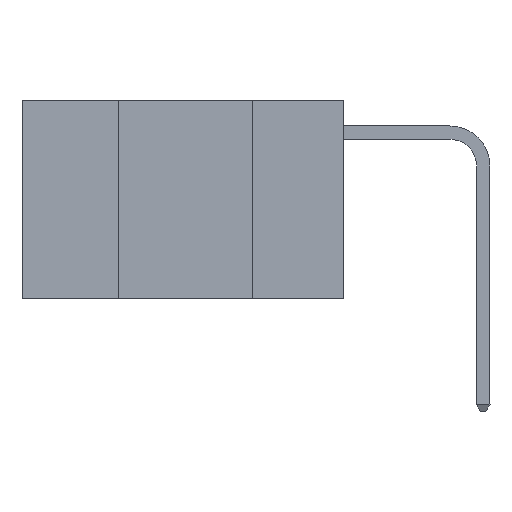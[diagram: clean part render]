
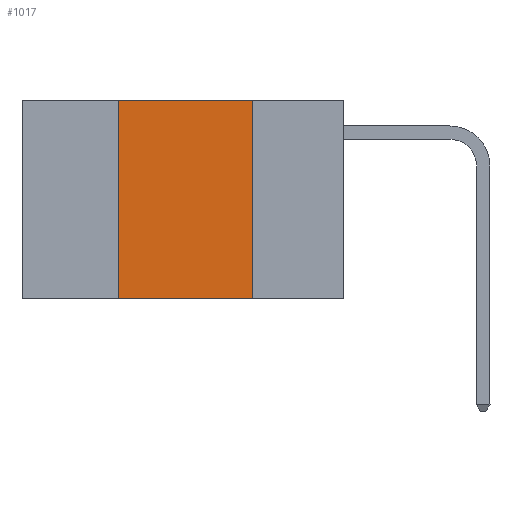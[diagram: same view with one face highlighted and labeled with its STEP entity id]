
A CAD part, left-side view. The second image highlights one B-rep face of the part: STEP entity #1017.
In plain terms, the highlighted planar face has unit normal (-1, 0, 0).
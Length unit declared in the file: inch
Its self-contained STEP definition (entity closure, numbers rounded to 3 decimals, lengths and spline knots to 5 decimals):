
#673 = ORIENTED_EDGE ( 'NONE', *, *, #3448, .F. ) ;
#968 = EDGE_CURVE ( 'NONE', #1902, #14417, #13548, .T. ) ;
#1017 = ADVANCED_FACE ( 'NONE', ( #9887 ), #10258, .F. ) ;
#1463 = VECTOR ( 'NONE', #7913, 39.37008 ) ;
#1902 = VERTEX_POINT ( 'NONE', #14021 ) ;
#2383 = LINE ( 'NONE', #5336, #5076 ) ;
#2518 = CARTESIAN_POINT ( 'NONE',  ( 0., 0.42, 0. ) ) ;
#3425 = DIRECTION ( 'NONE',  ( 1., 0., 0. ) ) ;
#3448 = EDGE_CURVE ( 'NONE', #1902, #10002, #7911, .T. ) ;
#4842 = VECTOR ( 'NONE', #9116, 39.37008 ) ;
#5076 = VECTOR ( 'NONE', #11002, 39.37008 ) ;
#5336 = CARTESIAN_POINT ( 'NONE',  ( 0., 0.6, 0. ) ) ;
#6303 = ORIENTED_EDGE ( 'NONE', *, *, #12049, .F. ) ;
#6387 = ORIENTED_EDGE ( 'NONE', *, *, #968, .T. ) ;
#7552 = LINE ( 'NONE', #14321, #13147 ) ;
#7606 = EDGE_CURVE ( 'NONE', #10962, #14417, #7552, .T. ) ;
#7911 = LINE ( 'NONE', #14645, #4842 ) ;
#7913 = DIRECTION ( 'NONE',  ( 0., -1., 0. ) ) ;
#7993 = EDGE_LOOP ( 'NONE', ( #13524, #6303, #673, #6387 ) ) ;
#8008 = CARTESIAN_POINT ( 'NONE',  ( 0., 0.6, 0. ) ) ;
#8070 = CARTESIAN_POINT ( 'NONE',  ( 0., 0.17, -0.37 ) ) ;
#9116 = DIRECTION ( 'NONE',  ( 0., 0., 1. ) ) ;
#9887 = FACE_OUTER_BOUND ( 'NONE', #7993, .T. ) ;
#10002 = VERTEX_POINT ( 'NONE', #2518 ) ;
#10258 = PLANE ( 'NONE',  #10731 ) ;
#10731 = AXIS2_PLACEMENT_3D ( 'NONE', #8008, #3425, #11369 ) ;
#10962 = VERTEX_POINT ( 'NONE', #14574 ) ;
#11002 = DIRECTION ( 'NONE',  ( 0., -1., 0. ) ) ;
#11016 = DIRECTION ( 'NONE',  ( 0., 0., -1. ) ) ;
#11369 = DIRECTION ( 'NONE',  ( 0., 0., -1. ) ) ;
#12049 = EDGE_CURVE ( 'NONE', #10002, #10962, #2383, .T. ) ;
#13147 = VECTOR ( 'NONE', #11016, 39.37008 ) ;
#13477 = CARTESIAN_POINT ( 'NONE',  ( 0., 0.6, -0.37 ) ) ;
#13524 = ORIENTED_EDGE ( 'NONE', *, *, #7606, .F. ) ;
#13548 = LINE ( 'NONE', #13477, #1463 ) ;
#14021 = CARTESIAN_POINT ( 'NONE',  ( 0., 0.42, -0.37 ) ) ;
#14321 = CARTESIAN_POINT ( 'NONE',  ( 0., 0.17, 0. ) ) ;
#14417 = VERTEX_POINT ( 'NONE', #8070 ) ;
#14574 = CARTESIAN_POINT ( 'NONE',  ( 0., 0.17, 0. ) ) ;
#14645 = CARTESIAN_POINT ( 'NONE',  ( 0., 0.42, 0. ) ) ;
